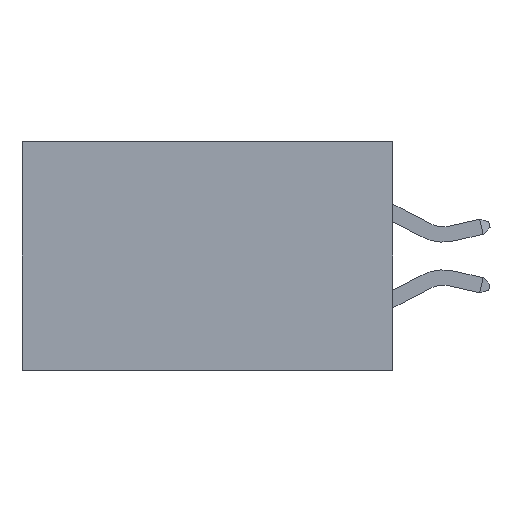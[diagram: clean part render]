
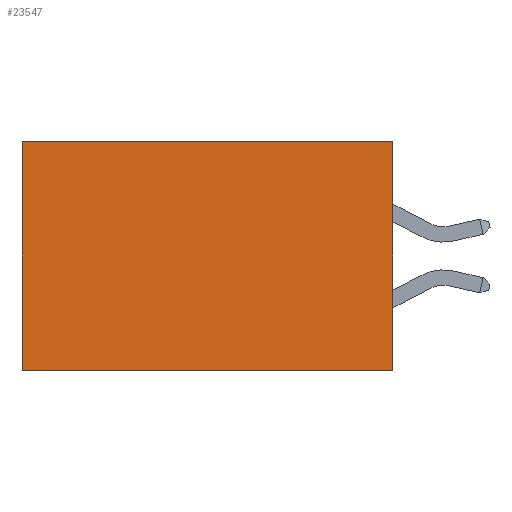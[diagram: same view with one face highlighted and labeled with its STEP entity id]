
A CAD part, left-side view. The second image highlights one B-rep face of the part: STEP entity #23547.
In plain terms, the highlighted planar face has unit normal (-1, 0, 0).
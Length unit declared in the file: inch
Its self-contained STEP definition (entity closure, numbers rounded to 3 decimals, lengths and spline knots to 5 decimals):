
#536 = ORIENTED_EDGE ( 'NONE', *, *, #1001, .T. ) ;
#886 = VERTEX_POINT ( 'NONE', #19674 ) ;
#1001 = EDGE_CURVE ( 'NONE', #2475, #886, #5072, .T. ) ;
#1670 = CARTESIAN_POINT ( 'NONE',  ( 0.2875, 0., 0. ) ) ;
#1818 = VERTEX_POINT ( 'NONE', #15333 ) ;
#2475 = VERTEX_POINT ( 'NONE', #2709 ) ;
#2709 = CARTESIAN_POINT ( 'NONE',  ( 0.2875, 0., 0. ) ) ;
#2722 = ORIENTED_EDGE ( 'NONE', *, *, #26408, .F. ) ;
#4483 = LINE ( 'NONE', #10756, #25404 ) ;
#4651 = EDGE_LOOP ( 'NONE', ( #18296, #14130, #2722, #536 ) ) ;
#5060 = PLANE ( 'NONE',  #23870 ) ;
#5072 = LINE ( 'NONE', #20045, #14842 ) ;
#5508 = LINE ( 'NONE', #1670, #26342 ) ;
#5914 = VERTEX_POINT ( 'NONE', #15285 ) ;
#7158 = DIRECTION ( 'NONE',  ( 0., 0., -1. ) ) ;
#8068 = DIRECTION ( 'NONE',  ( 0., 0., -1. ) ) ;
#8081 = FACE_OUTER_BOUND ( 'NONE', #4651, .T. ) ;
#8535 = LINE ( 'NONE', #24143, #23946 ) ;
#9909 = DIRECTION ( 'NONE',  ( 0., 1., 0. ) ) ;
#10756 = CARTESIAN_POINT ( 'NONE',  ( 0.2875, 0., -0.37 ) ) ;
#10757 = EDGE_CURVE ( 'NONE', #5914, #1818, #4483, .T. ) ;
#13031 = DIRECTION ( 'NONE',  ( 0., 1., 0. ) ) ;
#14130 = ORIENTED_EDGE ( 'NONE', *, *, #10757, .F. ) ;
#14842 = VECTOR ( 'NONE', #9909, 39.37008 ) ;
#15285 = CARTESIAN_POINT ( 'NONE',  ( 0.2875, 0., -0.37 ) ) ;
#15333 = CARTESIAN_POINT ( 'NONE',  ( 0.2875, 0.6, -0.37 ) ) ;
#18296 = ORIENTED_EDGE ( 'NONE', *, *, #25223, .T. ) ;
#19329 = CARTESIAN_POINT ( 'NONE',  ( 0.2875, 0., 0. ) ) ;
#19418 = DIRECTION ( 'NONE',  ( 1., 0., 0. ) ) ;
#19674 = CARTESIAN_POINT ( 'NONE',  ( 0.2875, 0.6, 0. ) ) ;
#20045 = CARTESIAN_POINT ( 'NONE',  ( 0.2875, 0., 0. ) ) ;
#23547 = ADVANCED_FACE ( 'NONE', ( #8081 ), #5060, .F. ) ;
#23870 = AXIS2_PLACEMENT_3D ( 'NONE', #19329, #19418, #7158 ) ;
#23946 = VECTOR ( 'NONE', #26029, 39.37008 ) ;
#24143 = CARTESIAN_POINT ( 'NONE',  ( 0.2875, 0.6, 0. ) ) ;
#25223 = EDGE_CURVE ( 'NONE', #886, #1818, #8535, .T. ) ;
#25404 = VECTOR ( 'NONE', #13031, 39.37008 ) ;
#26029 = DIRECTION ( 'NONE',  ( 0., 0., -1. ) ) ;
#26342 = VECTOR ( 'NONE', #8068, 39.37008 ) ;
#26408 = EDGE_CURVE ( 'NONE', #2475, #5914, #5508, .T. ) ;
